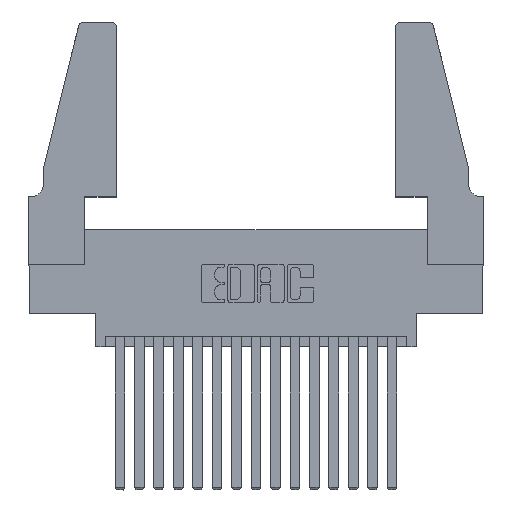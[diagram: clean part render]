
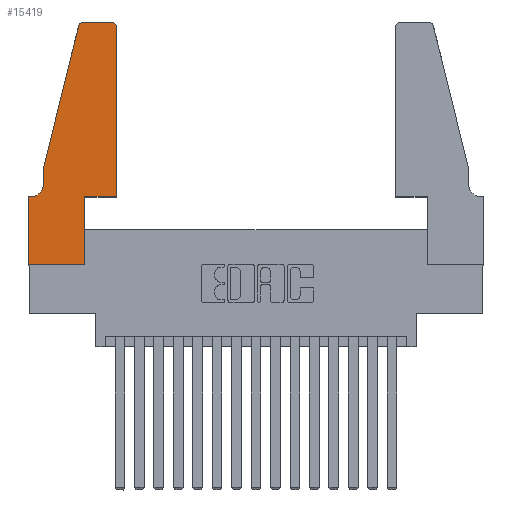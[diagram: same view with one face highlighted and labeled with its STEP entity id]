
A CAD part, top view. The second image highlights one B-rep face of the part: STEP entity #15419.
In plain terms, the highlighted planar face has unit normal (0, 0, 1).
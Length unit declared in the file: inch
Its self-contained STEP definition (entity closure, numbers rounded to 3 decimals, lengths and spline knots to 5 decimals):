
#71 = ORIENTED_EDGE ( 'NONE', *, *, #324, .T. ) ;
#213 = VERTEX_POINT ( 'NONE', #9735 ) ;
#290 = LINE ( 'NONE', #16109, #10202 ) ;
#324 = EDGE_CURVE ( 'NONE', #10468, #15438, #16657, .T. ) ;
#414 = EDGE_CURVE ( 'NONE', #8802, #213, #11103, .T. ) ;
#480 = FACE_OUTER_BOUND ( 'NONE', #3392, .T. ) ;
#681 = CARTESIAN_POINT ( 'NONE',  ( 0.2605, 1.25, 0.37 ) ) ;
#746 = VERTEX_POINT ( 'NONE', #12748 ) ;
#1014 = ORIENTED_EDGE ( 'NONE', *, *, #14484, .T. ) ;
#1173 = EDGE_CURVE ( 'NONE', #14978, #8802, #3049, .T. ) ;
#1218 = DIRECTION ( 'NONE',  ( 1., 0., 0. ) ) ;
#1396 = ORIENTED_EDGE ( 'NONE', *, *, #414, .T. ) ;
#1508 = VERTEX_POINT ( 'NONE', #10418 ) ;
#1612 = CARTESIAN_POINT ( 'NONE',  ( 0.0755, 0.5, 0.37 ) ) ;
#1723 = VERTEX_POINT ( 'NONE', #10040 ) ;
#1752 = CARTESIAN_POINT ( 'NONE',  ( 0., 0., 0.37 ) ) ;
#1905 = DIRECTION ( 'NONE',  ( 1., 0., 0. ) ) ;
#1953 = VERTEX_POINT ( 'NONE', #15465 ) ;
#2174 = AXIS2_PLACEMENT_3D ( 'NONE', #7692, #8998, #2489 ) ;
#2273 = VECTOR ( 'NONE', #1905, 39.37008 ) ;
#2371 = DIRECTION ( 'NONE',  ( 1., 0., 0. ) ) ;
#2489 = DIRECTION ( 'NONE',  ( 1., 0., 0. ) ) ;
#2586 = CIRCLE ( 'NONE', #9593, 0.03 ) ;
#3049 = LINE ( 'NONE', #4258, #12307 ) ;
#3392 = EDGE_LOOP ( 'NONE', ( #11852, #15212, #15781, #13520, #6994, #1014, #9129, #1396, #13713, #71, #12279, #13092 ) ) ;
#3587 = LINE ( 'NONE', #681, #8946 ) ;
#4114 = DIRECTION ( 'NONE',  ( -1., 0., 0. ) ) ;
#4258 = CARTESIAN_POINT ( 'NONE',  ( 0., 0., 0.37 ) ) ;
#4314 = CARTESIAN_POINT ( 'NONE',  ( 0.2865, 0.35, 0.37 ) ) ;
#4635 = DIRECTION ( 'NONE',  ( 1., 0., 0. ) ) ;
#5560 = LINE ( 'NONE', #13512, #9984 ) ;
#5582 = LINE ( 'NONE', #10343, #14922 ) ;
#6437 = CARTESIAN_POINT ( 'NONE',  ( 0.0755, 0.42, 0.37 ) ) ;
#6667 = EDGE_CURVE ( 'NONE', #1723, #746, #14071, .T. ) ;
#6994 = ORIENTED_EDGE ( 'NONE', *, *, #10385, .T. ) ;
#7210 = EDGE_CURVE ( 'NONE', #7749, #1953, #2586, .T. ) ;
#7692 = CARTESIAN_POINT ( 'NONE',  ( 0., 0.35, 0.37 ) ) ;
#7749 = VERTEX_POINT ( 'NONE', #15532 ) ;
#8130 = CARTESIAN_POINT ( 'NONE',  ( 0.0055, 0.42, 0.37 ) ) ;
#8244 = EDGE_CURVE ( 'NONE', #746, #7749, #3587, .T. ) ;
#8802 = VERTEX_POINT ( 'NONE', #1752 ) ;
#8946 = VECTOR ( 'NONE', #10050, 39.37008 ) ;
#8998 = DIRECTION ( 'NONE',  ( 0., 0., 1. ) ) ;
#9035 = LINE ( 'NONE', #1612, #12210 ) ;
#9056 = VECTOR ( 'NONE', #11478, 39.37008 ) ;
#9129 = ORIENTED_EDGE ( 'NONE', *, *, #1173, .T. ) ;
#9317 = DIRECTION ( 'NONE',  ( 0., 0., 1. ) ) ;
#9543 = VERTEX_POINT ( 'NONE', #6437 ) ;
#9593 = AXIS2_PLACEMENT_3D ( 'NONE', #10541, #11642, #2371 ) ;
#9666 = DIRECTION ( 'NONE',  ( -1., 0., 0. ) ) ;
#9735 = CARTESIAN_POINT ( 'NONE',  ( 0.2865, 0., 0.37 ) ) ;
#9857 = CARTESIAN_POINT ( 'NONE',  ( 0.4505, 0.35, 0.37 ) ) ;
#9984 = VECTOR ( 'NONE', #4114, 39.37008 ) ;
#10040 = CARTESIAN_POINT ( 'NONE',  ( 0.4505, 1.22, 0.37 ) ) ;
#10050 = DIRECTION ( 'NONE',  ( -1., 0., 0. ) ) ;
#10202 = VECTOR ( 'NONE', #17220, 39.37008 ) ;
#10328 = LINE ( 'NONE', #14255, #9056 ) ;
#10343 = CARTESIAN_POINT ( 'NONE',  ( 0.0755, 0.5, 0.37 ) ) ;
#10385 = EDGE_CURVE ( 'NONE', #9543, #1508, #17077, .T. ) ;
#10418 = CARTESIAN_POINT ( 'NONE',  ( 0.0055, 0.35, 0.37 ) ) ;
#10468 = VERTEX_POINT ( 'NONE', #4314 ) ;
#10541 = CARTESIAN_POINT ( 'NONE',  ( 0.284, 1.22, 0.37 ) ) ;
#10569 = CARTESIAN_POINT ( 'NONE',  ( 0., 0.35, 0.37 ) ) ;
#10729 = CARTESIAN_POINT ( 'NONE',  ( 0.4205, 1.22, 0.37 ) ) ;
#11103 = LINE ( 'NONE', #16425, #2273 ) ;
#11476 = EDGE_CURVE ( 'NONE', #1953, #12100, #5582, .T. ) ;
#11478 = DIRECTION ( 'NONE',  ( 0., 1., 0. ) ) ;
#11510 = VECTOR ( 'NONE', #4635, 39.37008 ) ;
#11642 = DIRECTION ( 'NONE',  ( 0., 0., 1. ) ) ;
#11685 = DIRECTION ( 'NONE',  ( -0.239, -0.971, 0. ) ) ;
#11852 = ORIENTED_EDGE ( 'NONE', *, *, #8244, .T. ) ;
#12098 = EDGE_CURVE ( 'NONE', #213, #10468, #290, .T. ) ;
#12100 = VERTEX_POINT ( 'NONE', #14557 ) ;
#12210 = VECTOR ( 'NONE', #12623, 39.37008 ) ;
#12256 = DIRECTION ( 'NONE',  ( 0., -1., 0. ) ) ;
#12279 = ORIENTED_EDGE ( 'NONE', *, *, #16690, .T. ) ;
#12307 = VECTOR ( 'NONE', #12256, 39.37008 ) ;
#12376 = DIRECTION ( 'NONE',  ( 0., 0., -1. ) ) ;
#12623 = DIRECTION ( 'NONE',  ( 0., -1., 0. ) ) ;
#12748 = CARTESIAN_POINT ( 'NONE',  ( 0.4205, 1.25, 0.37 ) ) ;
#13092 = ORIENTED_EDGE ( 'NONE', *, *, #6667, .T. ) ;
#13512 = CARTESIAN_POINT ( 'NONE',  ( 0.0755, 0.35, 0.37 ) ) ;
#13520 = ORIENTED_EDGE ( 'NONE', *, *, #17144, .T. ) ;
#13713 = ORIENTED_EDGE ( 'NONE', *, *, #12098, .T. ) ;
#14071 = CIRCLE ( 'NONE', #14609, 0.03 ) ;
#14255 = CARTESIAN_POINT ( 'NONE',  ( 0.4505, 0.35, 0.37 ) ) ;
#14413 = PLANE ( 'NONE',  #2174 ) ;
#14484 = EDGE_CURVE ( 'NONE', #1508, #14978, #5560, .T. ) ;
#14557 = CARTESIAN_POINT ( 'NONE',  ( 0.0755, 0.5, 0.37 ) ) ;
#14609 = AXIS2_PLACEMENT_3D ( 'NONE', #10729, #9317, #1218 ) ;
#14803 = AXIS2_PLACEMENT_3D ( 'NONE', #8130, #12376, #9666 ) ;
#14922 = VECTOR ( 'NONE', #11685, 39.37008 ) ;
#14978 = VERTEX_POINT ( 'NONE', #10569 ) ;
#15212 = ORIENTED_EDGE ( 'NONE', *, *, #7210, .T. ) ;
#15419 = ADVANCED_FACE ( 'NONE', ( #480 ), #14413, .T. ) ;
#15438 = VERTEX_POINT ( 'NONE', #17201 ) ;
#15465 = CARTESIAN_POINT ( 'NONE',  ( 0.25487, 1.22718, 0.37 ) ) ;
#15532 = CARTESIAN_POINT ( 'NONE',  ( 0.284, 1.25, 0.37 ) ) ;
#15781 = ORIENTED_EDGE ( 'NONE', *, *, #11476, .T. ) ;
#16109 = CARTESIAN_POINT ( 'NONE',  ( 0.2865, 0.35, 0.37 ) ) ;
#16425 = CARTESIAN_POINT ( 'NONE',  ( 0., 0., 0.37 ) ) ;
#16657 = LINE ( 'NONE', #9857, #11510 ) ;
#16690 = EDGE_CURVE ( 'NONE', #15438, #1723, #10328, .T. ) ;
#17077 = CIRCLE ( 'NONE', #14803, 0.07 ) ;
#17144 = EDGE_CURVE ( 'NONE', #12100, #9543, #9035, .T. ) ;
#17201 = CARTESIAN_POINT ( 'NONE',  ( 0.4505, 0.35, 0.37 ) ) ;
#17220 = DIRECTION ( 'NONE',  ( 0., 1., 0. ) ) ;
